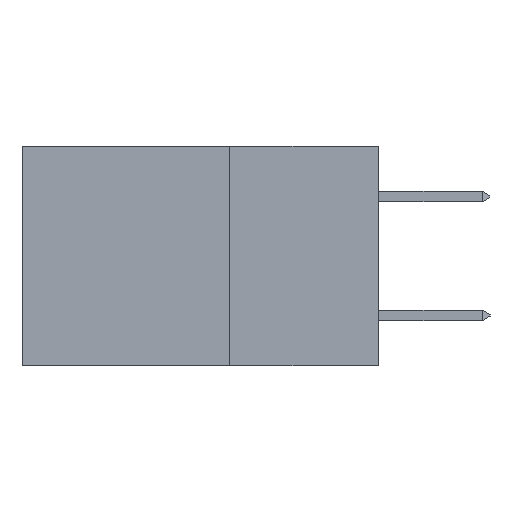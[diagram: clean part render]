
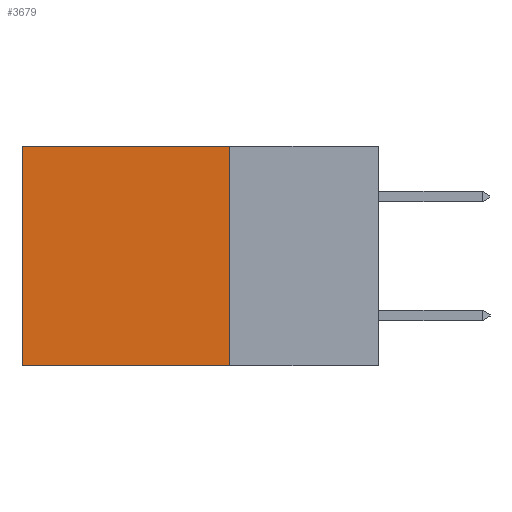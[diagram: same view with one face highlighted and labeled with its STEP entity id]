
A CAD part, left-side view. The second image highlights one B-rep face of the part: STEP entity #3679.
In plain terms, the highlighted planar face has unit normal (-1, 0, 0).
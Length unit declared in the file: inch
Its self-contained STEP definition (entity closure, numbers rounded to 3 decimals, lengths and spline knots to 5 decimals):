
#233 = DIRECTION ( 'NONE',  ( 0., 0., -1. ) ) ;
#1190 = CARTESIAN_POINT ( 'NONE',  ( 0.2615, 0.25, 0. ) ) ;
#1718 = FACE_OUTER_BOUND ( 'NONE', #3524, .T. ) ;
#1948 = VECTOR ( 'NONE', #233, 39.37008 ) ;
#1993 = LINE ( 'NONE', #7085, #4200 ) ;
#2163 = DIRECTION ( 'NONE',  ( 0., 0., -1. ) ) ;
#2205 = CARTESIAN_POINT ( 'NONE',  ( 0.2615, 0.25, -0.37 ) ) ;
#2311 = LINE ( 'NONE', #2205, #9095 ) ;
#2486 = CARTESIAN_POINT ( 'NONE',  ( 0.2615, 0.25, -0.37 ) ) ;
#2682 = VERTEX_POINT ( 'NONE', #2486 ) ;
#2747 = EDGE_CURVE ( 'NONE', #4882, #2682, #2311, .T. ) ;
#2960 = DIRECTION ( 'NONE',  ( 0., 1., 0. ) ) ;
#2976 = CARTESIAN_POINT ( 'NONE',  ( 0.2615, 0.6, -0.37 ) ) ;
#3039 = CARTESIAN_POINT ( 'NONE',  ( 0.2615, 0.6, -0.37 ) ) ;
#3053 = DIRECTION ( 'NONE',  ( 0., 1., 0. ) ) ;
#3188 = VERTEX_POINT ( 'NONE', #11298 ) ;
#3524 = EDGE_LOOP ( 'NONE', ( #5111, #5355, #5402, #5415 ) ) ;
#3679 = ADVANCED_FACE ( 'NONE', ( #1718 ), #6470, .F. ) ;
#3899 = CARTESIAN_POINT ( 'NONE',  ( 0.2615, 0.25, 0. ) ) ;
#4123 = AXIS2_PLACEMENT_3D ( 'NONE', #6217, #4285, #4253 ) ;
#4162 = EDGE_CURVE ( 'NONE', #2682, #4364, #1993, .T. ) ;
#4200 = VECTOR ( 'NONE', #3053, 39.37008 ) ;
#4253 = DIRECTION ( 'NONE',  ( 0., 0., -1. ) ) ;
#4285 = DIRECTION ( 'NONE',  ( 1., 0., 0. ) ) ;
#4364 = VERTEX_POINT ( 'NONE', #2976 ) ;
#4882 = VERTEX_POINT ( 'NONE', #1190 ) ;
#4884 = EDGE_CURVE ( 'NONE', #3188, #4364, #9611, .T. ) ;
#5111 = ORIENTED_EDGE ( 'NONE', *, *, #4884, .T. ) ;
#5355 = ORIENTED_EDGE ( 'NONE', *, *, #4162, .F. ) ;
#5402 = ORIENTED_EDGE ( 'NONE', *, *, #2747, .F. ) ;
#5415 = ORIENTED_EDGE ( 'NONE', *, *, #6738, .T. ) ;
#6217 = CARTESIAN_POINT ( 'NONE',  ( 0.2615, 0.25, -0.37 ) ) ;
#6449 = LINE ( 'NONE', #3899, #11037 ) ;
#6470 = PLANE ( 'NONE',  #4123 ) ;
#6738 = EDGE_CURVE ( 'NONE', #4882, #3188, #6449, .T. ) ;
#7085 = CARTESIAN_POINT ( 'NONE',  ( 0.2615, 0.25, -0.37 ) ) ;
#9095 = VECTOR ( 'NONE', #2163, 39.37008 ) ;
#9611 = LINE ( 'NONE', #3039, #1948 ) ;
#11037 = VECTOR ( 'NONE', #2960, 39.37008 ) ;
#11298 = CARTESIAN_POINT ( 'NONE',  ( 0.2615, 0.6, 0. ) ) ;
